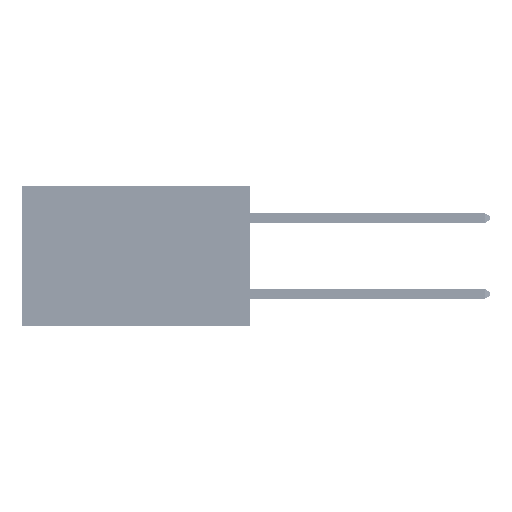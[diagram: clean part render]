
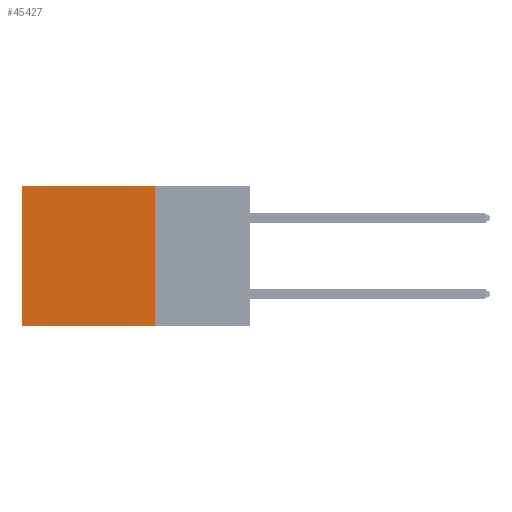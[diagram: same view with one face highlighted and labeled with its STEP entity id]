
A CAD part, left-side view. The second image highlights one B-rep face of the part: STEP entity #45427.
In plain terms, the highlighted planar face has unit normal (-1, 0, 0).
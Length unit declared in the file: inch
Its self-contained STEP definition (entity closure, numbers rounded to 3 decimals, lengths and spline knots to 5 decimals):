
#1038 = AXIS2_PLACEMENT_3D ( 'NONE', #44609, #40760, #44453 ) ;
#1194 = EDGE_CURVE ( 'NONE', #45944, #9489, #12234, .T. ) ;
#2371 = DIRECTION ( 'NONE',  ( 0., 1., 0. ) ) ;
#3688 = EDGE_CURVE ( 'NONE', #27440, #34025, #24735, .T. ) ;
#6203 = DIRECTION ( 'NONE',  ( 0., 0., -1. ) ) ;
#8843 = VECTOR ( 'NONE', #32165, 39.37008 ) ;
#9045 = ORIENTED_EDGE ( 'NONE', *, *, #3688, .F. ) ;
#9489 = VERTEX_POINT ( 'NONE', #47937 ) ;
#9716 = CARTESIAN_POINT ( 'NONE',  ( 0.2875, 0.25, 0. ) ) ;
#12234 = LINE ( 'NONE', #14129, #18854 ) ;
#12463 = ORIENTED_EDGE ( 'NONE', *, *, #29312, .T. ) ;
#14129 = CARTESIAN_POINT ( 'NONE',  ( 0.2875, 0.6, 0. ) ) ;
#14133 = FACE_OUTER_BOUND ( 'NONE', #44069, .T. ) ;
#16117 = LINE ( 'NONE', #28931, #8843 ) ;
#16519 = ORIENTED_EDGE ( 'NONE', *, *, #1194, .T. ) ;
#18854 = VECTOR ( 'NONE', #6203, 39.37008 ) ;
#24735 = LINE ( 'NONE', #49886, #42147 ) ;
#25298 = PLANE ( 'NONE',  #1038 ) ;
#25510 = CARTESIAN_POINT ( 'NONE',  ( 0.2875, 0.25, -0.37 ) ) ;
#27440 = VERTEX_POINT ( 'NONE', #9716 ) ;
#28931 = CARTESIAN_POINT ( 'NONE',  ( 0.2875, 0.25, 0. ) ) ;
#29312 = EDGE_CURVE ( 'NONE', #27440, #45944, #16117, .T. ) ;
#32165 = DIRECTION ( 'NONE',  ( 0., 1., 0. ) ) ;
#32863 = CARTESIAN_POINT ( 'NONE',  ( 0.2875, 0.25, -0.37 ) ) ;
#34025 = VERTEX_POINT ( 'NONE', #32863 ) ;
#35814 = LINE ( 'NONE', #25510, #44808 ) ;
#39143 = ORIENTED_EDGE ( 'NONE', *, *, #46776, .F. ) ;
#40373 = CARTESIAN_POINT ( 'NONE',  ( 0.2875, 0.6, 0. ) ) ;
#40760 = DIRECTION ( 'NONE',  ( 1., 0., 0. ) ) ;
#42147 = VECTOR ( 'NONE', #45853, 39.37008 ) ;
#44069 = EDGE_LOOP ( 'NONE', ( #16519, #39143, #9045, #12463 ) ) ;
#44453 = DIRECTION ( 'NONE',  ( 0., 0., -1. ) ) ;
#44609 = CARTESIAN_POINT ( 'NONE',  ( 0.2875, 0.25, 0. ) ) ;
#44808 = VECTOR ( 'NONE', #2371, 39.37008 ) ;
#45427 = ADVANCED_FACE ( 'NONE', ( #14133 ), #25298, .F. ) ;
#45853 = DIRECTION ( 'NONE',  ( 0., 0., -1. ) ) ;
#45944 = VERTEX_POINT ( 'NONE', #40373 ) ;
#46776 = EDGE_CURVE ( 'NONE', #34025, #9489, #35814, .T. ) ;
#47937 = CARTESIAN_POINT ( 'NONE',  ( 0.2875, 0.6, -0.37 ) ) ;
#49886 = CARTESIAN_POINT ( 'NONE',  ( 0.2875, 0.25, 0. ) ) ;
